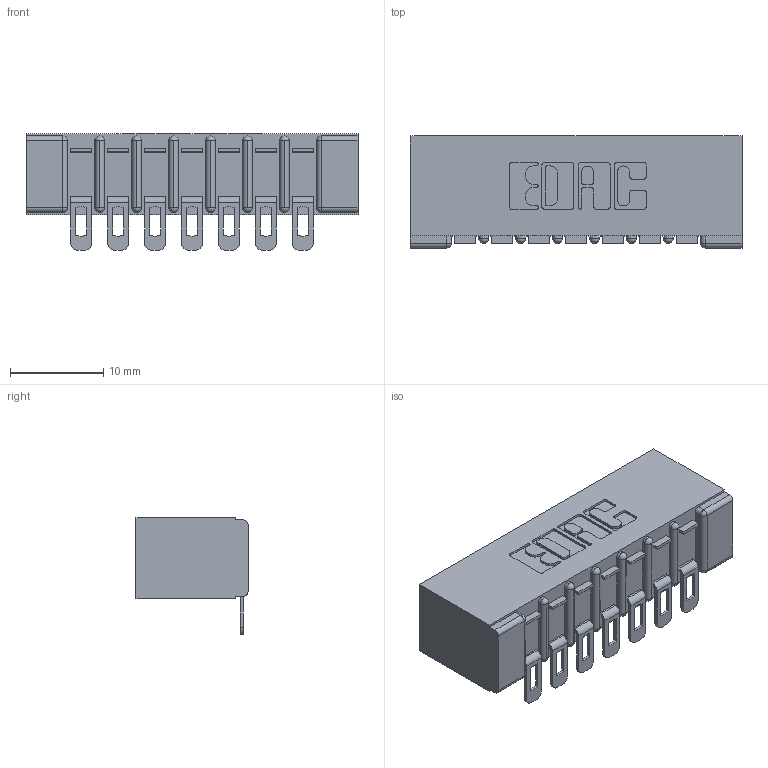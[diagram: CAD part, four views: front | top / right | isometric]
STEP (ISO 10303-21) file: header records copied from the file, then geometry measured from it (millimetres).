
FILE_DESCRIPTION (( 'STEP AP203' ), '1' );
FILE_NAME ('357-007-454-101.STEP', '2020-09-30T02:35:08', ( '' ), ( '' ), 'SwSTEP 2.0', 'SolidWorks 2020', '' );
FILE_SCHEMA (( 'CONFIG_CONTROL_DESIGN' ));
Length unit declared in the file: inch
Products named in the file (3): 307 Part_No Mounting Lugs; 357-007-454-101; 307-290-002_554
Assembly tree (8 placements, depth 2):
  357-007-454-101
    307 Part_No Mounting Lugs
    307-290-002_554  x7
Bounding box: 35.61 x 12.01 x 12.52 mm (x, y, z)
Volume: 2587.9 mm3; surface area: 4409 mm2
Topology: 8 solids, 8 shells, 685 faces, 2070 edges, 1356 vertices
Faces by surface type: plane 388, cylinder 281, sphere 16
Entity records: 11003 total; most frequent: CARTESIAN_POINT 1850, ORIENTED_EDGE 1840, DIRECTION 1818, EDGE_CURVE 920, LINE 682, VECTOR 682, VERTEX_POINT 600, AXIS2_PLACEMENT_3D 568
